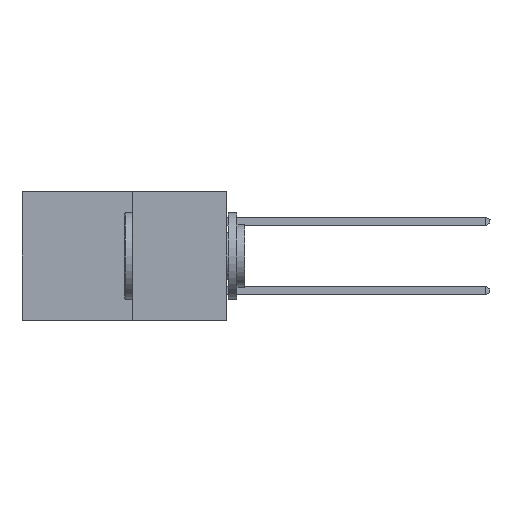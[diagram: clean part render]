
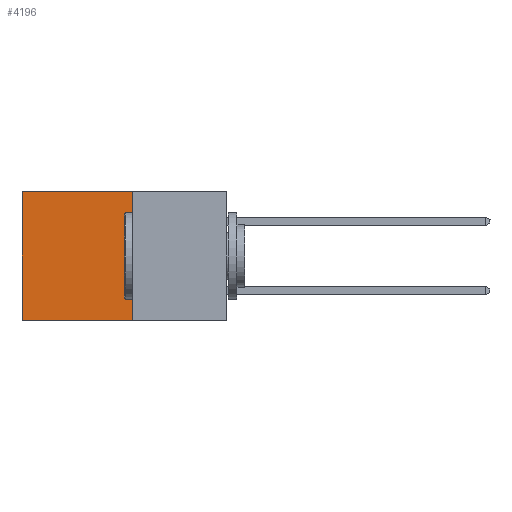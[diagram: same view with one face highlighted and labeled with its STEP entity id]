
A CAD part, left-side view. The second image highlights one B-rep face of the part: STEP entity #4196.
In plain terms, the highlighted planar face has unit normal (-1, 0, 0).
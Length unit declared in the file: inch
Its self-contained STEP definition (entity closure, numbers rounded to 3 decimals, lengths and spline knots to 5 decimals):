
#15 = ORIENTED_EDGE ( 'NONE', *, *, #1070, .F. ) ;
#26 = VECTOR ( 'NONE', #8883, 39.37008 ) ;
#157 = VECTOR ( 'NONE', #3307, 39.37008 ) ;
#228 = EDGE_CURVE ( 'NONE', #7109, #3725, #8256, .T. ) ;
#481 = EDGE_CURVE ( 'NONE', #7109, #6814, #2806, .T. ) ;
#1070 = EDGE_CURVE ( 'NONE', #3725, #4221, #4789, .T. ) ;
#2448 = CARTESIAN_POINT ( 'NONE',  ( 0.277, 0.59, -0.37 ) ) ;
#2529 = ORIENTED_EDGE ( 'NONE', *, *, #228, .F. ) ;
#2806 = LINE ( 'NONE', #8226, #26 ) ;
#2903 = CARTESIAN_POINT ( 'NONE',  ( 0.277, 0.59, -0.37 ) ) ;
#2945 = FACE_OUTER_BOUND ( 'NONE', #8834, .T. ) ;
#3047 = DIRECTION ( 'NONE',  ( 0., 0., -1. ) ) ;
#3051 = DIRECTION ( 'NONE',  ( 1., 0., 0. ) ) ;
#3063 = CARTESIAN_POINT ( 'NONE',  ( 0.277, 0.27, -0.37 ) ) ;
#3174 = PLANE ( 'NONE',  #6925 ) ;
#3307 = DIRECTION ( 'NONE',  ( 0., 1., 0. ) ) ;
#3725 = VERTEX_POINT ( 'NONE', #4639 ) ;
#4196 = ADVANCED_FACE ( 'NONE', ( #2945 ), #3174, .F. ) ;
#4221 = VERTEX_POINT ( 'NONE', #2903 ) ;
#4544 = CARTESIAN_POINT ( 'NONE',  ( 0.277, 0.27, -0.37 ) ) ;
#4639 = CARTESIAN_POINT ( 'NONE',  ( 0.277, 0.27, -0.37 ) ) ;
#4789 = LINE ( 'NONE', #4544, #157 ) ;
#4850 = CARTESIAN_POINT ( 'NONE',  ( 0.277, 0.27, -0.37 ) ) ;
#5264 = VECTOR ( 'NONE', #8564, 39.37008 ) ;
#6006 = ORIENTED_EDGE ( 'NONE', *, *, #7926, .T. ) ;
#6196 = ORIENTED_EDGE ( 'NONE', *, *, #481, .T. ) ;
#6681 = VECTOR ( 'NONE', #7201, 39.37008 ) ;
#6814 = VERTEX_POINT ( 'NONE', #6860 ) ;
#6860 = CARTESIAN_POINT ( 'NONE',  ( 0.277, 0.59, 0. ) ) ;
#6925 = AXIS2_PLACEMENT_3D ( 'NONE', #3063, #3051, #3047 ) ;
#7109 = VERTEX_POINT ( 'NONE', #8056 ) ;
#7201 = DIRECTION ( 'NONE',  ( 0., 0., -1. ) ) ;
#7926 = EDGE_CURVE ( 'NONE', #6814, #4221, #8760, .T. ) ;
#8056 = CARTESIAN_POINT ( 'NONE',  ( 0.277, 0.27, 0. ) ) ;
#8226 = CARTESIAN_POINT ( 'NONE',  ( 0.277, 0.27, 0. ) ) ;
#8256 = LINE ( 'NONE', #4850, #5264 ) ;
#8564 = DIRECTION ( 'NONE',  ( 0., 0., -1. ) ) ;
#8760 = LINE ( 'NONE', #2448, #6681 ) ;
#8834 = EDGE_LOOP ( 'NONE', ( #6006, #15, #2529, #6196 ) ) ;
#8883 = DIRECTION ( 'NONE',  ( 0., 1., 0. ) ) ;
